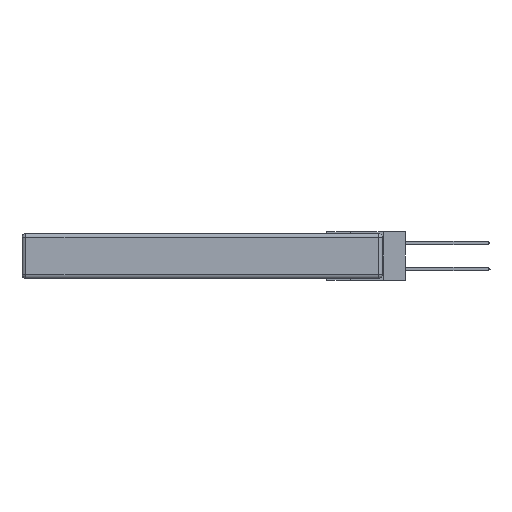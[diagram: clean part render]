
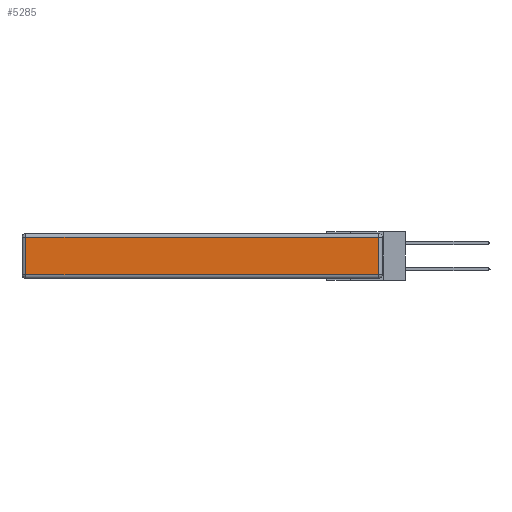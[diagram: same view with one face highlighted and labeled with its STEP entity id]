
A CAD part, left-side view. The second image highlights one B-rep face of the part: STEP entity #5285.
In plain terms, the highlighted planar face has unit normal (-1, 0, 0).
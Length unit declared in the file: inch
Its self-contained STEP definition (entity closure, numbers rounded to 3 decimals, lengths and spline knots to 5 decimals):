
#361 = LINE ( 'NONE', #4085, #4763 ) ;
#728 = DIRECTION ( 'NONE',  ( 0., 0., -1. ) ) ;
#1174 = EDGE_LOOP ( 'NONE', ( #12130, #13305, #7915, #10301 ) ) ;
#1239 = CARTESIAN_POINT ( 'NONE',  ( 0., 0.03, -0.343 ) ) ;
#1814 = LINE ( 'NONE', #12547, #12603 ) ;
#1882 = DIRECTION ( 'NONE',  ( -1., 0., 0. ) ) ;
#3516 = AXIS2_PLACEMENT_3D ( 'NONE', #13351, #1882, #9209 ) ;
#3600 = CARTESIAN_POINT ( 'NONE',  ( 0., 2.72, -0.03 ) ) ;
#4085 = CARTESIAN_POINT ( 'NONE',  ( 0., 0., -0.313 ) ) ;
#4282 = VERTEX_POINT ( 'NONE', #12974 ) ;
#4763 = VECTOR ( 'NONE', #8413, 39.37008 ) ;
#4992 = VECTOR ( 'NONE', #6379, 39.37008 ) ;
#5285 = ADVANCED_FACE ( 'NONE', ( #10230 ), #10236, .T. ) ;
#6237 = EDGE_CURVE ( 'NONE', #10706, #4282, #10362, .T. ) ;
#6379 = DIRECTION ( 'NONE',  ( 0., 0., 1. ) ) ;
#6750 = EDGE_CURVE ( 'NONE', #9297, #10323, #11685, .T. ) ;
#7915 = ORIENTED_EDGE ( 'NONE', *, *, #12484, .T. ) ;
#8413 = DIRECTION ( 'NONE',  ( 0., -1., 0. ) ) ;
#9209 = DIRECTION ( 'NONE',  ( 0., 0., 1. ) ) ;
#9297 = VERTEX_POINT ( 'NONE', #3600 ) ;
#10192 = VECTOR ( 'NONE', #728, 39.37008 ) ;
#10230 = FACE_OUTER_BOUND ( 'NONE', #1174, .T. ) ;
#10236 = PLANE ( 'NONE',  #3516 ) ;
#10301 = ORIENTED_EDGE ( 'NONE', *, *, #6750, .T. ) ;
#10323 = VERTEX_POINT ( 'NONE', #12749 ) ;
#10362 = LINE ( 'NONE', #1239, #4992 ) ;
#10706 = VERTEX_POINT ( 'NONE', #13056 ) ;
#11471 = DIRECTION ( 'NONE',  ( 0., 1., 0. ) ) ;
#11685 = LINE ( 'NONE', #13265, #10192 ) ;
#12130 = ORIENTED_EDGE ( 'NONE', *, *, #12914, .T. ) ;
#12484 = EDGE_CURVE ( 'NONE', #4282, #9297, #1814, .T. ) ;
#12547 = CARTESIAN_POINT ( 'NONE',  ( 0., 2.75, -0.03 ) ) ;
#12603 = VECTOR ( 'NONE', #11471, 39.37008 ) ;
#12749 = CARTESIAN_POINT ( 'NONE',  ( 0., 2.72, -0.313 ) ) ;
#12914 = EDGE_CURVE ( 'NONE', #10323, #10706, #361, .T. ) ;
#12974 = CARTESIAN_POINT ( 'NONE',  ( 0., 0.03, -0.03 ) ) ;
#13056 = CARTESIAN_POINT ( 'NONE',  ( 0., 0.03, -0.313 ) ) ;
#13265 = CARTESIAN_POINT ( 'NONE',  ( 0., 2.72, -0.343 ) ) ;
#13305 = ORIENTED_EDGE ( 'NONE', *, *, #6237, .T. ) ;
#13351 = CARTESIAN_POINT ( 'NONE',  ( 0., 0., -0.343 ) ) ;
